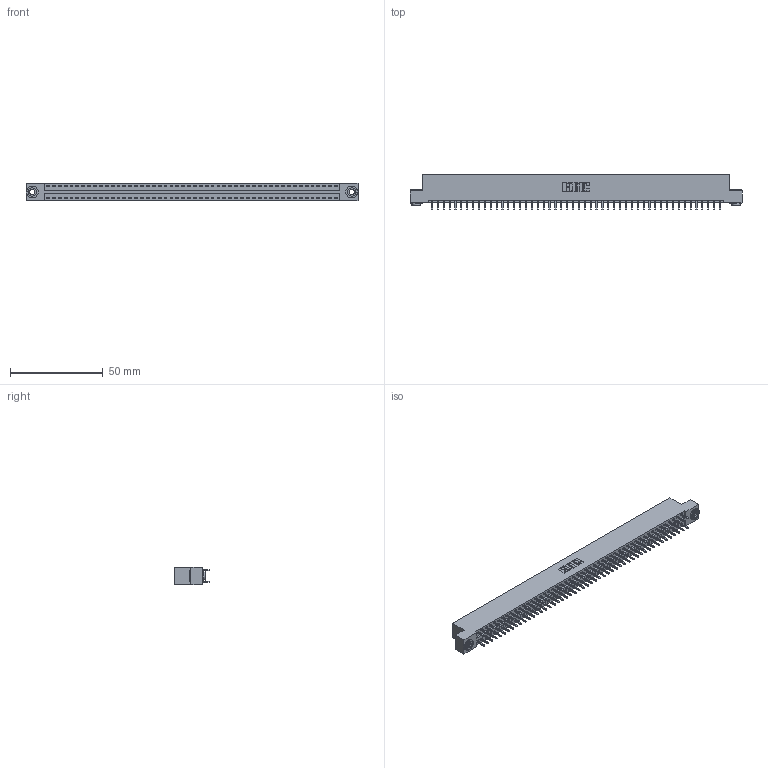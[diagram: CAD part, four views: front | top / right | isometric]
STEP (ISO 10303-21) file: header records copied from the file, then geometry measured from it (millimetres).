
FILE_DESCRIPTION (( 'STEP AP203' ), '1' );
FILE_NAME ('396-100-521-203.STEP', '2018-09-14T06:36:50', ( '' ), ( '' ), 'SwSTEP 2.0', 'SolidWorks 2016', '' );
FILE_SCHEMA (( 'CONFIG_CONTROL_DESIGN' ));
Length unit declared in the file: inch
Products named in the file (4): 346 Part_Flush Mounting Lugs - 0.156 Dia-TH; 345-292-001_345-293-121; 345-250-002_345-250-002-102; 396-100-521-203
Assembly tree (103 placements, depth 2):
  396-100-521-203
    346 Part_Flush Mounting Lugs - 0.156 Dia-TH
    345-292-001_345-293-121  x100
    345-250-002_345-250-002-102  x2
Bounding box: 179.32 x 19.05 x 9.4 mm (x, y, z)
Volume: 17527 mm3; surface area: 24157.2 mm2
Topology: 103 solids, 103 shells, 5360 faces, 15905 edges, 10466 vertices
Faces by surface type: plane 3586, cylinder 1766, cone 8
Entity records: 32222 total; most frequent: CARTESIAN_POINT 5275, ORIENTED_EDGE 5202, DIRECTION 4731, EDGE_CURVE 2601, LINE 2245, VECTOR 2245, VERTEX_POINT 1730, AXIS2_PLACEMENT_3D 1243
